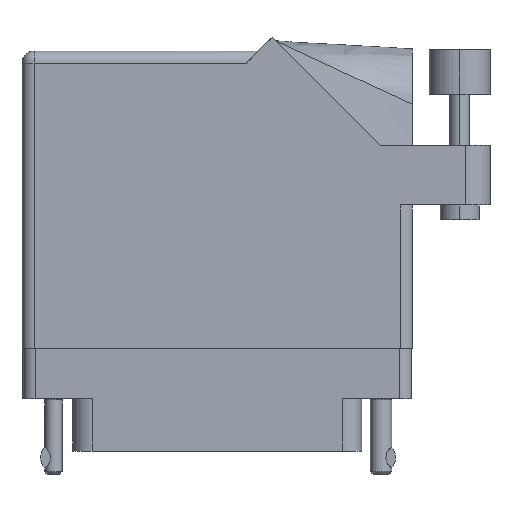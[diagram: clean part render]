
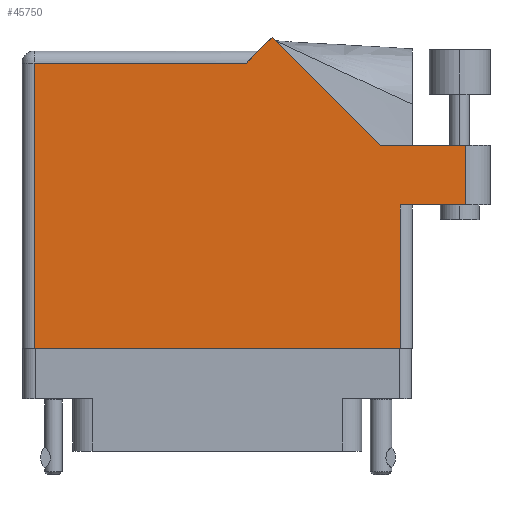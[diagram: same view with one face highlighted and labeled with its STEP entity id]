
A CAD part, front view. The second image highlights one B-rep face of the part: STEP entity #45750.
In plain terms, the highlighted face is planar.
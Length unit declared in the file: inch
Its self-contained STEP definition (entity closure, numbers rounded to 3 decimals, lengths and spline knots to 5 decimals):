
#1733 = VERTEX_POINT ( 'NONE', #4997 ) ;
#2504 = VERTEX_POINT ( 'NONE', #25601 ) ;
#2689 = DIRECTION ( 'NONE',  ( -0.707, -0.707, 0. ) ) ;
#2900 = VERTEX_POINT ( 'NONE', #22209 ) ;
#4035 = VERTEX_POINT ( 'NONE', #10587 ) ;
#4622 = CARTESIAN_POINT ( 'NONE',  ( 2.285, 1.044, 0. ) ) ;
#4725 = DIRECTION ( 'NONE',  ( -0.707, 0.707, 0. ) ) ;
#4997 = CARTESIAN_POINT ( 'NONE',  ( 1.155, 1.468, 0. ) ) ;
#5245 = CARTESIAN_POINT ( 'NONE',  ( 0., 1.53, 0. ) ) ;
#6072 = LINE ( 'NONE', #46908, #15989 ) ;
#7729 = ORIENTED_EDGE ( 'NONE', *, *, #37286, .T. ) ;
#8166 = CARTESIAN_POINT ( 'NONE',  ( 1.84442, 1.044, 0. ) ) ;
#8422 = EDGE_CURVE ( 'NONE', #2900, #35329, #38317, .T. ) ;
#10077 = VECTOR ( 'NONE', #4725, 39.37008 ) ;
#10587 = CARTESIAN_POINT ( 'NONE',  ( 2.285, 0.737, 0. ) ) ;
#10697 = VECTOR ( 'NONE', #15320, 39.37008 ) ;
#10730 = VERTEX_POINT ( 'NONE', #11298 ) ;
#10843 = EDGE_CURVE ( 'NONE', #26169, #4035, #12568, .T. ) ;
#11298 = CARTESIAN_POINT ( 'NONE',  ( 1.948, 0., 0. ) ) ;
#11576 = ORIENTED_EDGE ( 'NONE', *, *, #24946, .T. ) ;
#12568 = LINE ( 'NONE', #14657, #28822 ) ;
#14042 = VECTOR ( 'NONE', #2689, 39.37008 ) ;
#14604 = ORIENTED_EDGE ( 'NONE', *, *, #37577, .T. ) ;
#14607 = CARTESIAN_POINT ( 'NONE',  ( 1.948, 0.737, 0. ) ) ;
#14657 = CARTESIAN_POINT ( 'NONE',  ( 2.01, 0.737, 0. ) ) ;
#15320 = DIRECTION ( 'NONE',  ( 0., 1., 0. ) ) ;
#15601 = CARTESIAN_POINT ( 'NONE',  ( 2.285, 1.044, 0. ) ) ;
#15908 = LINE ( 'NONE', #45385, #10697 ) ;
#15989 = VECTOR ( 'NONE', #47385, 39.37008 ) ;
#16068 = AXIS2_PLACEMENT_3D ( 'NONE', #5245, #31905, #27555 ) ;
#16462 = LINE ( 'NONE', #8166, #10077 ) ;
#17386 = EDGE_CURVE ( 'NONE', #2504, #1733, #18070, .T. ) ;
#18070 = LINE ( 'NONE', #32622, #14042 ) ;
#18184 = LINE ( 'NONE', #15601, #21087 ) ;
#19486 = DIRECTION ( 'NONE',  ( 0., -1., 0. ) ) ;
#19503 = VERTEX_POINT ( 'NONE', #4622 ) ;
#20338 = ORIENTED_EDGE ( 'NONE', *, *, #17386, .T. ) ;
#21087 = VECTOR ( 'NONE', #41264, 39.37008 ) ;
#22008 = CARTESIAN_POINT ( 'NONE',  ( 1.84442, 1.044, 0. ) ) ;
#22209 = CARTESIAN_POINT ( 'NONE',  ( 0.062, 1.468, 0. ) ) ;
#23605 = LINE ( 'NONE', #45142, #38701 ) ;
#24946 = EDGE_CURVE ( 'NONE', #35329, #10730, #23605, .T. ) ;
#25042 = DIRECTION ( 'NONE',  ( -1., 0., 0. ) ) ;
#25601 = CARTESIAN_POINT ( 'NONE',  ( 1.28771, 1.60071, 0. ) ) ;
#26169 = VERTEX_POINT ( 'NONE', #14607 ) ;
#27555 = DIRECTION ( 'NONE',  ( -1., 0., 0. ) ) ;
#27855 = PLANE ( 'NONE',  #16068 ) ;
#28821 = VERTEX_POINT ( 'NONE', #22008 ) ;
#28822 = VECTOR ( 'NONE', #33327, 39.37008 ) ;
#29506 = ORIENTED_EDGE ( 'NONE', *, *, #10843, .T. ) ;
#30793 = EDGE_LOOP ( 'NONE', ( #29506, #47806, #47983, #7729, #20338, #14604, #39310, #11576, #35824 ) ) ;
#31905 = DIRECTION ( 'NONE',  ( 0., 0., -1. ) ) ;
#32622 = CARTESIAN_POINT ( 'NONE',  ( 1.217, 1.53, 0. ) ) ;
#33327 = DIRECTION ( 'NONE',  ( 1., 0., 0. ) ) ;
#34563 = DIRECTION ( 'NONE',  ( 1., 0., 0. ) ) ;
#35329 = VERTEX_POINT ( 'NONE', #46137 ) ;
#35824 = ORIENTED_EDGE ( 'NONE', *, *, #46041, .T. ) ;
#35957 = EDGE_CURVE ( 'NONE', #19503, #28821, #6072, .T. ) ;
#37286 = EDGE_CURVE ( 'NONE', #28821, #2504, #16462, .T. ) ;
#37577 = EDGE_CURVE ( 'NONE', #1733, #2900, #47852, .T. ) ;
#37806 = EDGE_CURVE ( 'NONE', #4035, #19503, #18184, .T. ) ;
#37842 = CARTESIAN_POINT ( 'NONE',  ( 0.062, 0., 0. ) ) ;
#37925 = VECTOR ( 'NONE', #25042, 39.37008 ) ;
#38317 = LINE ( 'NONE', #37842, #44159 ) ;
#38701 = VECTOR ( 'NONE', #34563, 39.37008 ) ;
#39310 = ORIENTED_EDGE ( 'NONE', *, *, #8422, .T. ) ;
#41264 = DIRECTION ( 'NONE',  ( 0., 1., 0. ) ) ;
#44159 = VECTOR ( 'NONE', #19486, 39.37008 ) ;
#45142 = CARTESIAN_POINT ( 'NONE',  ( 0., 0., 0. ) ) ;
#45385 = CARTESIAN_POINT ( 'NONE',  ( 1.948, 0.737, 0. ) ) ;
#45750 = ADVANCED_FACE ( 'NONE', ( #46762 ), #27855, .F. ) ;
#46041 = EDGE_CURVE ( 'NONE', #10730, #26169, #15908, .T. ) ;
#46137 = CARTESIAN_POINT ( 'NONE',  ( 0.062, 0., 0. ) ) ;
#46762 = FACE_OUTER_BOUND ( 'NONE', #30793, .T. ) ;
#46908 = CARTESIAN_POINT ( 'NONE',  ( 2.41, 1.044, 0. ) ) ;
#47385 = DIRECTION ( 'NONE',  ( -1., 0., 0. ) ) ;
#47495 = CARTESIAN_POINT ( 'NONE',  ( 0., 1.468, 0. ) ) ;
#47806 = ORIENTED_EDGE ( 'NONE', *, *, #37806, .T. ) ;
#47852 = LINE ( 'NONE', #47495, #37925 ) ;
#47983 = ORIENTED_EDGE ( 'NONE', *, *, #35957, .T. ) ;
